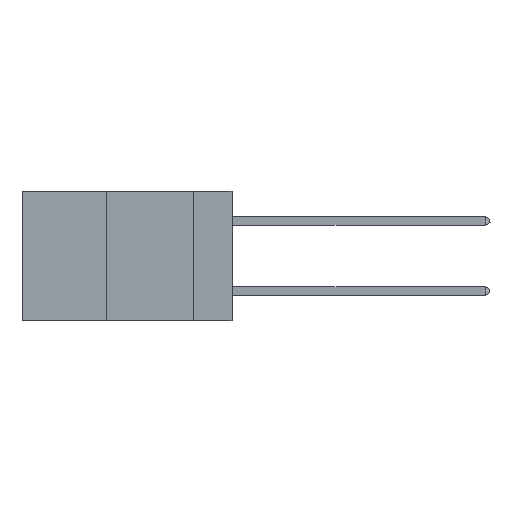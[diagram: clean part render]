
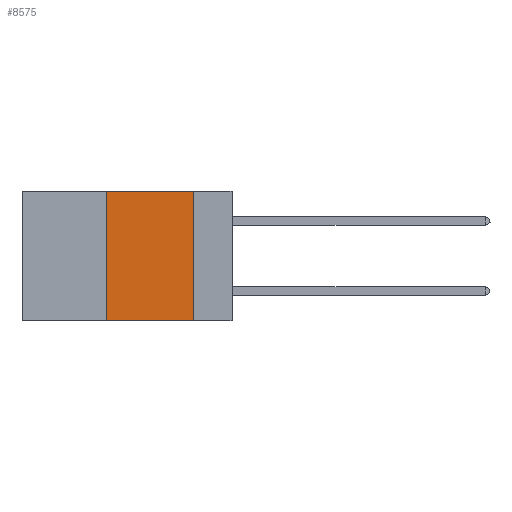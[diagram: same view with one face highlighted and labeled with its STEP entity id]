
A CAD part, left-side view. The second image highlights one B-rep face of the part: STEP entity #8575.
In plain terms, the highlighted planar face has unit normal (-1, 0, 0).
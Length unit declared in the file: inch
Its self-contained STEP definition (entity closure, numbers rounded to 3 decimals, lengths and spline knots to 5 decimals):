
#3 = LINE ( 'NONE', #14858, #8954 ) ;
#812 = ORIENTED_EDGE ( 'NONE', *, *, #11820, .T. ) ;
#1077 = VERTEX_POINT ( 'NONE', #14644 ) ;
#1647 = PLANE ( 'NONE',  #10733 ) ;
#1899 = VERTEX_POINT ( 'NONE', #11473 ) ;
#2039 = LINE ( 'NONE', #7882, #16323 ) ;
#2316 = DIRECTION ( 'NONE',  ( 0., 0., 1. ) ) ;
#2537 = CARTESIAN_POINT ( 'NONE',  ( 0., 0.6, 0. ) ) ;
#4151 = LINE ( 'NONE', #2537, #16262 ) ;
#4297 = DIRECTION ( 'NONE',  ( 0., -1., 0. ) ) ;
#5068 = LINE ( 'NONE', #14294, #12968 ) ;
#6992 = DIRECTION ( 'NONE',  ( 0., 0., -1. ) ) ;
#7459 = VERTEX_POINT ( 'NONE', #9396 ) ;
#7882 = CARTESIAN_POINT ( 'NONE',  ( 0., 0.6, -0.37 ) ) ;
#8575 = ADVANCED_FACE ( 'NONE', ( #21427 ), #1647, .F. ) ;
#8954 = VECTOR ( 'NONE', #2316, 39.37008 ) ;
#9396 = CARTESIAN_POINT ( 'NONE',  ( 0., 0.36, 0. ) ) ;
#9895 = ORIENTED_EDGE ( 'NONE', *, *, #21894, .F. ) ;
#10288 = ORIENTED_EDGE ( 'NONE', *, *, #21807, .F. ) ;
#10733 = AXIS2_PLACEMENT_3D ( 'NONE', #19482, #17756, #6992 ) ;
#10985 = VERTEX_POINT ( 'NONE', #14772 ) ;
#11315 = EDGE_LOOP ( 'NONE', ( #15269, #9895, #10288, #812 ) ) ;
#11473 = CARTESIAN_POINT ( 'NONE',  ( 0., 0.36, -0.37 ) ) ;
#11523 = EDGE_CURVE ( 'NONE', #10985, #1077, #5068, .T. ) ;
#11820 = EDGE_CURVE ( 'NONE', #1899, #1077, #2039, .T. ) ;
#12968 = VECTOR ( 'NONE', #16083, 39.37008 ) ;
#14294 = CARTESIAN_POINT ( 'NONE',  ( 0., 0.11, 0. ) ) ;
#14644 = CARTESIAN_POINT ( 'NONE',  ( 0., 0.11, -0.37 ) ) ;
#14772 = CARTESIAN_POINT ( 'NONE',  ( 0., 0.11, 0. ) ) ;
#14858 = CARTESIAN_POINT ( 'NONE',  ( 0., 0.36, 0. ) ) ;
#15269 = ORIENTED_EDGE ( 'NONE', *, *, #11523, .F. ) ;
#16083 = DIRECTION ( 'NONE',  ( 0., 0., -1. ) ) ;
#16262 = VECTOR ( 'NONE', #4297, 39.37008 ) ;
#16323 = VECTOR ( 'NONE', #22166, 39.37008 ) ;
#17756 = DIRECTION ( 'NONE',  ( 1., 0., 0. ) ) ;
#19482 = CARTESIAN_POINT ( 'NONE',  ( 0., 0.6, 0. ) ) ;
#21427 = FACE_OUTER_BOUND ( 'NONE', #11315, .T. ) ;
#21807 = EDGE_CURVE ( 'NONE', #1899, #7459, #3, .T. ) ;
#21894 = EDGE_CURVE ( 'NONE', #7459, #10985, #4151, .T. ) ;
#22166 = DIRECTION ( 'NONE',  ( 0., -1., 0. ) ) ;
